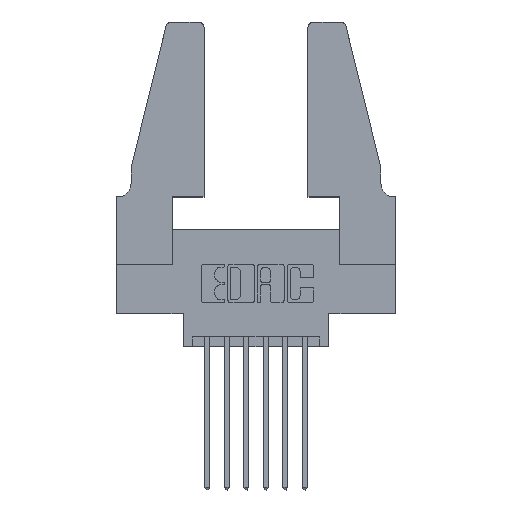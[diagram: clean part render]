
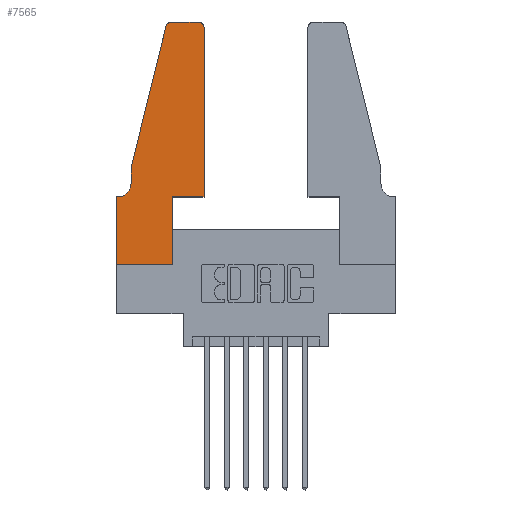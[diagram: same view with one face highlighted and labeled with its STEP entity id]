
A CAD part, top view. The second image highlights one B-rep face of the part: STEP entity #7565.
In plain terms, the highlighted planar face has unit normal (0, 0, 1).
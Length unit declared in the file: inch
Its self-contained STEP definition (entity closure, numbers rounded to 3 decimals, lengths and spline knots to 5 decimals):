
#193 = AXIS2_PLACEMENT_3D ( 'NONE', #9406, #3939, #10319 ) ;
#269 = DIRECTION ( 'NONE',  ( 0., 0., 1. ) ) ;
#438 = ORIENTED_EDGE ( 'NONE', *, *, #10412, .T. ) ;
#510 = LINE ( 'NONE', #6902, #7542 ) ;
#724 = VECTOR ( 'NONE', #5050, 39.37008 ) ;
#725 = LINE ( 'NONE', #8928, #9614 ) ;
#878 = EDGE_CURVE ( 'NONE', #8523, #4693, #9624, .T. ) ;
#1016 = LINE ( 'NONE', #1262, #724 ) ;
#1071 = ORIENTED_EDGE ( 'NONE', *, *, #1270, .T. ) ;
#1075 = ORIENTED_EDGE ( 'NONE', *, *, #4875, .T. ) ;
#1185 = CIRCLE ( 'NONE', #193, 0.03 ) ;
#1262 = CARTESIAN_POINT ( 'NONE',  ( 0., 0., 0.37 ) ) ;
#1270 = EDGE_CURVE ( 'NONE', #2827, #8523, #1016, .T. ) ;
#1456 = CARTESIAN_POINT ( 'NONE',  ( 0.2865, 0., 0.37 ) ) ;
#1487 = VECTOR ( 'NONE', #4685, 39.37008 ) ;
#1669 = ORIENTED_EDGE ( 'NONE', *, *, #5870, .T. ) ;
#2164 = ORIENTED_EDGE ( 'NONE', *, *, #10484, .T. ) ;
#2250 = CARTESIAN_POINT ( 'NONE',  ( 0., 0.35, 0.37 ) ) ;
#2275 = CARTESIAN_POINT ( 'NONE',  ( 0.4205, 1.25, 0.37 ) ) ;
#2384 = DIRECTION ( 'NONE',  ( -0.239, -0.971, 0. ) ) ;
#2517 = VERTEX_POINT ( 'NONE', #7784 ) ;
#2827 = VERTEX_POINT ( 'NONE', #10402 ) ;
#2851 = DIRECTION ( 'NONE',  ( 0., -1., 0. ) ) ;
#2900 = VERTEX_POINT ( 'NONE', #9530 ) ;
#3013 = ORIENTED_EDGE ( 'NONE', *, *, #6761, .T. ) ;
#3050 = ORIENTED_EDGE ( 'NONE', *, *, #3335, .T. ) ;
#3131 = DIRECTION ( 'NONE',  ( 0., 0., -1. ) ) ;
#3263 = VECTOR ( 'NONE', #5834, 39.37008 ) ;
#3335 = EDGE_CURVE ( 'NONE', #9066, #9250, #10277, .T. ) ;
#3450 = AXIS2_PLACEMENT_3D ( 'NONE', #5821, #269, #6746 ) ;
#3492 = VERTEX_POINT ( 'NONE', #4580 ) ;
#3789 = CARTESIAN_POINT ( 'NONE',  ( 0.2865, 0.35, 0.37 ) ) ;
#3916 = VECTOR ( 'NONE', #2851, 39.37008 ) ;
#3939 = DIRECTION ( 'NONE',  ( 0., 0., 1. ) ) ;
#4036 = CARTESIAN_POINT ( 'NONE',  ( 0.4505, 0.35, 0.37 ) ) ;
#4087 = VERTEX_POINT ( 'NONE', #8459 ) ;
#4428 = VECTOR ( 'NONE', #5589, 39.37008 ) ;
#4430 = EDGE_CURVE ( 'NONE', #2517, #5941, #725, .T. ) ;
#4548 = DIRECTION ( 'NONE',  ( 0., 0., 1. ) ) ;
#4580 = CARTESIAN_POINT ( 'NONE',  ( 0.0755, 0.42, 0.37 ) ) ;
#4685 = DIRECTION ( 'NONE',  ( 0., -1., 0. ) ) ;
#4693 = VERTEX_POINT ( 'NONE', #3789 ) ;
#4875 = EDGE_CURVE ( 'NONE', #4693, #2517, #10164, .T. ) ;
#4877 = CARTESIAN_POINT ( 'NONE',  ( 0.25487, 1.22718, 0.37 ) ) ;
#4950 = VERTEX_POINT ( 'NONE', #2250 ) ;
#4980 = AXIS2_PLACEMENT_3D ( 'NONE', #10022, #4548, #10939 ) ;
#5050 = DIRECTION ( 'NONE',  ( 1., 0., 0. ) ) ;
#5172 = EDGE_LOOP ( 'NONE', ( #3050, #2164, #11353, #438, #3013, #1669, #6832, #1071, #7030, #1075, #7432, #5332 ) ) ;
#5327 = VECTOR ( 'NONE', #10422, 39.37008 ) ;
#5332 = ORIENTED_EDGE ( 'NONE', *, *, #11155, .T. ) ;
#5589 = DIRECTION ( 'NONE',  ( -1., 0., 0. ) ) ;
#5675 = DIRECTION ( 'NONE',  ( 0., 1., 0. ) ) ;
#5815 = CARTESIAN_POINT ( 'NONE',  ( 0.2605, 1.25, 0.37 ) ) ;
#5821 = CARTESIAN_POINT ( 'NONE',  ( 0.4205, 1.22, 0.37 ) ) ;
#5834 = DIRECTION ( 'NONE',  ( -1., 0., 0. ) ) ;
#5870 = EDGE_CURVE ( 'NONE', #4087, #4950, #11410, .T. ) ;
#5941 = VERTEX_POINT ( 'NONE', #10189 ) ;
#6299 = AXIS2_PLACEMENT_3D ( 'NONE', #8654, #3131, #9546 ) ;
#6746 = DIRECTION ( 'NONE',  ( 1., 0., 0. ) ) ;
#6761 = EDGE_CURVE ( 'NONE', #3492, #4087, #7135, .T. ) ;
#6832 = ORIENTED_EDGE ( 'NONE', *, *, #8842, .T. ) ;
#6902 = CARTESIAN_POINT ( 'NONE',  ( 0.0755, 0.5, 0.37 ) ) ;
#7030 = ORIENTED_EDGE ( 'NONE', *, *, #878, .T. ) ;
#7122 = DIRECTION ( 'NONE',  ( 0., 1., 0. ) ) ;
#7135 = CIRCLE ( 'NONE', #6299, 0.07 ) ;
#7432 = ORIENTED_EDGE ( 'NONE', *, *, #4430, .T. ) ;
#7457 = CARTESIAN_POINT ( 'NONE',  ( 0.0755, 0.5, 0.37 ) ) ;
#7542 = VECTOR ( 'NONE', #2384, 39.37008 ) ;
#7565 = ADVANCED_FACE ( 'NONE', ( #11239 ), #10898, .T. ) ;
#7784 = CARTESIAN_POINT ( 'NONE',  ( 0.4505, 0.35, 0.37 ) ) ;
#7865 = EDGE_CURVE ( 'NONE', #11187, #2900, #510, .T. ) ;
#8459 = CARTESIAN_POINT ( 'NONE',  ( 0.0055, 0.35, 0.37 ) ) ;
#8523 = VERTEX_POINT ( 'NONE', #1456 ) ;
#8654 = CARTESIAN_POINT ( 'NONE',  ( 0.0055, 0.42, 0.37 ) ) ;
#8842 = EDGE_CURVE ( 'NONE', #4950, #2827, #10918, .T. ) ;
#8928 = CARTESIAN_POINT ( 'NONE',  ( 0.4505, 0.35, 0.37 ) ) ;
#9066 = VERTEX_POINT ( 'NONE', #2275 ) ;
#9229 = CARTESIAN_POINT ( 'NONE',  ( 0.2865, 0.35, 0.37 ) ) ;
#9250 = VERTEX_POINT ( 'NONE', #10727 ) ;
#9406 = CARTESIAN_POINT ( 'NONE',  ( 0.284, 1.22, 0.37 ) ) ;
#9530 = CARTESIAN_POINT ( 'NONE',  ( 0.0755, 0.5, 0.37 ) ) ;
#9546 = DIRECTION ( 'NONE',  ( -1., 0., 0. ) ) ;
#9614 = VECTOR ( 'NONE', #7122, 39.37008 ) ;
#9624 = LINE ( 'NONE', #9229, #11454 ) ;
#9887 = CIRCLE ( 'NONE', #3450, 0.03 ) ;
#10022 = CARTESIAN_POINT ( 'NONE',  ( 0., 0.35, 0.37 ) ) ;
#10164 = LINE ( 'NONE', #4036, #5327 ) ;
#10189 = CARTESIAN_POINT ( 'NONE',  ( 0.4505, 1.22, 0.37 ) ) ;
#10277 = LINE ( 'NONE', #5815, #3263 ) ;
#10319 = DIRECTION ( 'NONE',  ( 1., 0., 0. ) ) ;
#10402 = CARTESIAN_POINT ( 'NONE',  ( 0., 0., 0.37 ) ) ;
#10412 = EDGE_CURVE ( 'NONE', #2900, #3492, #11183, .T. ) ;
#10422 = DIRECTION ( 'NONE',  ( 1., 0., 0. ) ) ;
#10484 = EDGE_CURVE ( 'NONE', #9250, #11187, #1185, .T. ) ;
#10727 = CARTESIAN_POINT ( 'NONE',  ( 0.284, 1.25, 0.37 ) ) ;
#10898 = PLANE ( 'NONE',  #4980 ) ;
#10918 = LINE ( 'NONE', #11070, #1487 ) ;
#10939 = DIRECTION ( 'NONE',  ( 1., 0., 0. ) ) ;
#11024 = CARTESIAN_POINT ( 'NONE',  ( 0.0755, 0.35, 0.37 ) ) ;
#11070 = CARTESIAN_POINT ( 'NONE',  ( 0., 0., 0.37 ) ) ;
#11155 = EDGE_CURVE ( 'NONE', #5941, #9066, #9887, .T. ) ;
#11183 = LINE ( 'NONE', #7457, #3916 ) ;
#11187 = VERTEX_POINT ( 'NONE', #4877 ) ;
#11239 = FACE_OUTER_BOUND ( 'NONE', #5172, .T. ) ;
#11353 = ORIENTED_EDGE ( 'NONE', *, *, #7865, .T. ) ;
#11410 = LINE ( 'NONE', #11024, #4428 ) ;
#11454 = VECTOR ( 'NONE', #5675, 39.37008 ) ;
